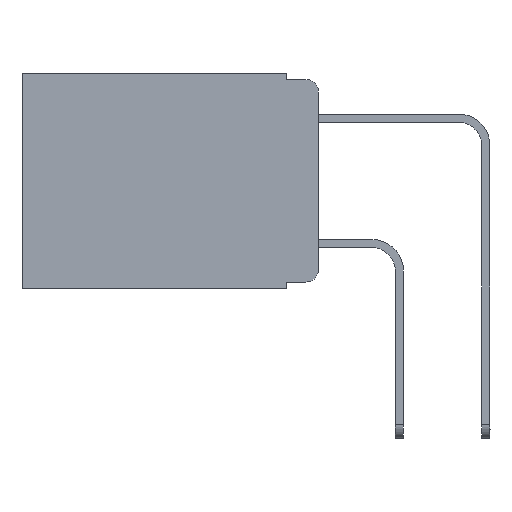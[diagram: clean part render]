
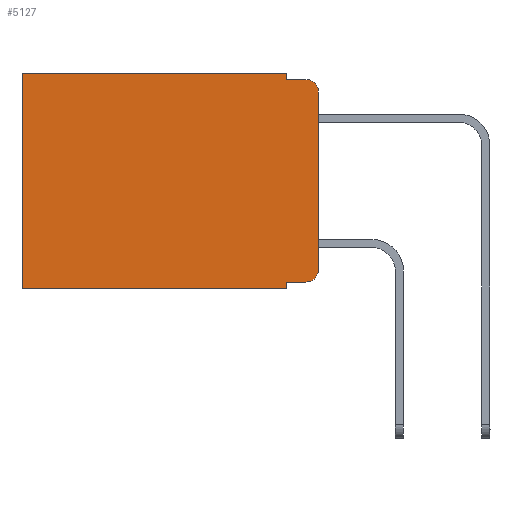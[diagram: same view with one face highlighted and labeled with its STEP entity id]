
A CAD part, left-side view. The second image highlights one B-rep face of the part: STEP entity #5127.
In plain terms, the highlighted planar face has unit normal (-1, 0, 0).
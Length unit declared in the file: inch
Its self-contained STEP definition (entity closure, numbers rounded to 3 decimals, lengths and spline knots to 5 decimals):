
#85 = DIRECTION ( 'NONE',  ( 0., -1., 0. ) ) ;
#745 = LINE ( 'NONE', #19214, #4578 ) ;
#1097 = VECTOR ( 'NONE', #85, 39.37008 ) ;
#1100 = LINE ( 'NONE', #12961, #19406 ) ;
#1190 = ORIENTED_EDGE ( 'NONE', *, *, #4793, .F. ) ;
#1754 = CARTESIAN_POINT ( 'NONE',  ( 0.298, 0.051, -0.01 ) ) ;
#1897 = LINE ( 'NONE', #9321, #23460 ) ;
#2281 = AXIS2_PLACEMENT_3D ( 'NONE', #8473, #13889, #5056 ) ;
#2409 = LINE ( 'NONE', #18539, #1097 ) ;
#2487 = DIRECTION ( 'NONE',  ( 0., 0., -1. ) ) ;
#2610 = CARTESIAN_POINT ( 'NONE',  ( 0.298, 0.051, 0. ) ) ;
#2664 = EDGE_CURVE ( 'NONE', #21689, #6564, #1100, .T. ) ;
#2783 = EDGE_CURVE ( 'NONE', #2848, #5264, #7657, .T. ) ;
#2806 = DIRECTION ( 'NONE',  ( 0., 0., -1. ) ) ;
#2848 = VERTEX_POINT ( 'NONE', #23282 ) ;
#2958 = DIRECTION ( 'NONE',  ( 0., 0., -1. ) ) ;
#2971 = EDGE_CURVE ( 'NONE', #5264, #23079, #3019, .T. ) ;
#3019 = LINE ( 'NONE', #10427, #14393 ) ;
#3964 = DIRECTION ( 'NONE',  ( 0., 1., 0. ) ) ;
#3968 = CIRCLE ( 'NONE', #22563, 0.02 ) ;
#4552 = DIRECTION ( 'NONE',  ( 0., -1., 0. ) ) ;
#4560 = LINE ( 'NONE', #2610, #11348 ) ;
#4578 = VECTOR ( 'NONE', #4552, 39.37008 ) ;
#4793 = EDGE_CURVE ( 'NONE', #7404, #14003, #1897, .T. ) ;
#5056 = DIRECTION ( 'NONE',  ( 0., 0., -1. ) ) ;
#5127 = ADVANCED_FACE ( 'NONE', ( #6885 ), #14254, .F. ) ;
#5264 = VERTEX_POINT ( 'NONE', #22587 ) ;
#5823 = CARTESIAN_POINT ( 'NONE',  ( 0.298, 0., 0. ) ) ;
#6471 = EDGE_CURVE ( 'NONE', #7404, #14244, #3968, .T. ) ;
#6564 = VERTEX_POINT ( 'NONE', #20532 ) ;
#6715 = EDGE_CURVE ( 'NONE', #21689, #8965, #745, .T. ) ;
#6885 = FACE_OUTER_BOUND ( 'NONE', #16587, .T. ) ;
#7112 = ORIENTED_EDGE ( 'NONE', *, *, #6715, .T. ) ;
#7404 = VERTEX_POINT ( 'NONE', #9214 ) ;
#7657 = LINE ( 'NONE', #5823, #19798 ) ;
#8399 = ORIENTED_EDGE ( 'NONE', *, *, #15109, .F. ) ;
#8473 = CARTESIAN_POINT ( 'NONE',  ( 0.298, 0., 0. ) ) ;
#8600 = DIRECTION ( 'NONE',  ( 0., 0., -1. ) ) ;
#8855 = EDGE_CURVE ( 'NONE', #8965, #14003, #15447, .T. ) ;
#8965 = VERTEX_POINT ( 'NONE', #14066 ) ;
#9214 = CARTESIAN_POINT ( 'NONE',  ( 0.298, 0., -0.03 ) ) ;
#9271 = EDGE_CURVE ( 'NONE', #12718, #14244, #2409, .T. ) ;
#9321 = CARTESIAN_POINT ( 'NONE',  ( 0.298, 0., 0. ) ) ;
#9439 = DIRECTION ( 'NONE',  ( 0., 0., -1. ) ) ;
#10281 = ORIENTED_EDGE ( 'NONE', *, *, #9271, .F. ) ;
#10427 = CARTESIAN_POINT ( 'NONE',  ( 0.298, 0.473, 0. ) ) ;
#11348 = VECTOR ( 'NONE', #2487, 39.37008 ) ;
#12008 = CARTESIAN_POINT ( 'NONE',  ( 0.298, 0.02, -0.313 ) ) ;
#12138 = DIRECTION ( 'NONE',  ( -1., 0., 0. ) ) ;
#12214 = CARTESIAN_POINT ( 'NONE',  ( 0.298, 0.02, -0.03 ) ) ;
#12718 = VERTEX_POINT ( 'NONE', #1754 ) ;
#12961 = CARTESIAN_POINT ( 'NONE',  ( 0.298, 0.051, 0. ) ) ;
#13153 = LINE ( 'NONE', #20552, #21453 ) ;
#13889 = DIRECTION ( 'NONE',  ( 1., 0., 0. ) ) ;
#14003 = VERTEX_POINT ( 'NONE', #22798 ) ;
#14066 = CARTESIAN_POINT ( 'NONE',  ( 0.298, 0.02, -0.333 ) ) ;
#14244 = VERTEX_POINT ( 'NONE', #19750 ) ;
#14254 = PLANE ( 'NONE',  #2281 ) ;
#14393 = VECTOR ( 'NONE', #19384, 39.37008 ) ;
#15050 = CARTESIAN_POINT ( 'NONE',  ( 0.298, 0.473, -0.343 ) ) ;
#15109 = EDGE_CURVE ( 'NONE', #2848, #12718, #4560, .T. ) ;
#15447 = CIRCLE ( 'NONE', #20096, 0.02 ) ;
#16587 = EDGE_LOOP ( 'NONE', ( #1190, #18240, #10281, #8399, #22624, #19037, #17284, #19262, #7112, #18069 ) ) ;
#17284 = ORIENTED_EDGE ( 'NONE', *, *, #17774, .F. ) ;
#17774 = EDGE_CURVE ( 'NONE', #6564, #23079, #13153, .T. ) ;
#18069 = ORIENTED_EDGE ( 'NONE', *, *, #8855, .T. ) ;
#18240 = ORIENTED_EDGE ( 'NONE', *, *, #6471, .T. ) ;
#18539 = CARTESIAN_POINT ( 'NONE',  ( 0.298, 0.051, -0.01 ) ) ;
#19037 = ORIENTED_EDGE ( 'NONE', *, *, #2971, .T. ) ;
#19148 = CARTESIAN_POINT ( 'NONE',  ( 0.298, 0.051, -0.333 ) ) ;
#19214 = CARTESIAN_POINT ( 'NONE',  ( 0.298, 0.051, -0.333 ) ) ;
#19262 = ORIENTED_EDGE ( 'NONE', *, *, #2664, .F. ) ;
#19384 = DIRECTION ( 'NONE',  ( 0., 0., -1. ) ) ;
#19406 = VECTOR ( 'NONE', #2958, 39.37008 ) ;
#19713 = DIRECTION ( 'NONE',  ( -1., 0., 0. ) ) ;
#19750 = CARTESIAN_POINT ( 'NONE',  ( 0.298, 0.02, -0.01 ) ) ;
#19798 = VECTOR ( 'NONE', #22681, 39.37008 ) ;
#20096 = AXIS2_PLACEMENT_3D ( 'NONE', #12008, #12138, #2806 ) ;
#20532 = CARTESIAN_POINT ( 'NONE',  ( 0.298, 0.051, -0.343 ) ) ;
#20552 = CARTESIAN_POINT ( 'NONE',  ( 0.298, 0., -0.343 ) ) ;
#21453 = VECTOR ( 'NONE', #3964, 39.37008 ) ;
#21689 = VERTEX_POINT ( 'NONE', #19148 ) ;
#22563 = AXIS2_PLACEMENT_3D ( 'NONE', #12214, #19713, #8600 ) ;
#22587 = CARTESIAN_POINT ( 'NONE',  ( 0.298, 0.473, 0. ) ) ;
#22624 = ORIENTED_EDGE ( 'NONE', *, *, #2783, .T. ) ;
#22681 = DIRECTION ( 'NONE',  ( 0., 1., 0. ) ) ;
#22798 = CARTESIAN_POINT ( 'NONE',  ( 0.298, 0., -0.313 ) ) ;
#23079 = VERTEX_POINT ( 'NONE', #15050 ) ;
#23282 = CARTESIAN_POINT ( 'NONE',  ( 0.298, 0.051, 0. ) ) ;
#23460 = VECTOR ( 'NONE', #9439, 39.37008 ) ;
